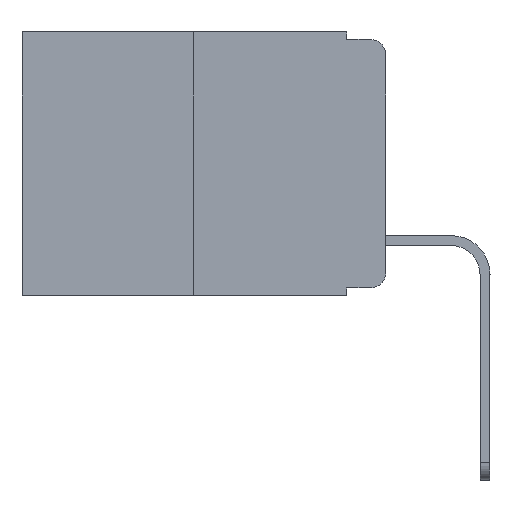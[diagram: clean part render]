
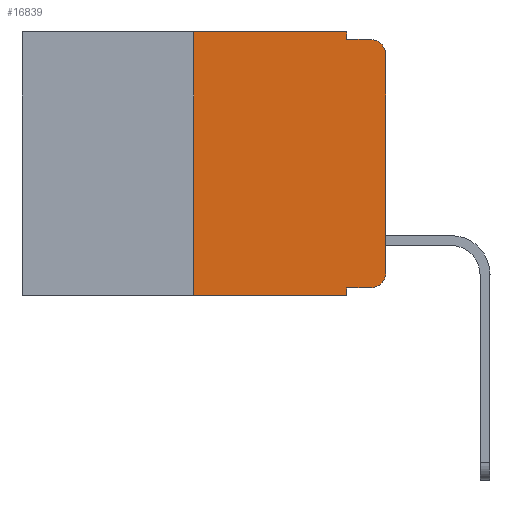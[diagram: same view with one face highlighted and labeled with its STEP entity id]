
A CAD part, left-side view. The second image highlights one B-rep face of the part: STEP entity #16839.
In plain terms, the highlighted planar face has unit normal (-1, 0, 0).
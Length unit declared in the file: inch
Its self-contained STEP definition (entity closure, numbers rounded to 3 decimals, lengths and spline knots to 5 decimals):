
#220 = ORIENTED_EDGE ( 'NONE', *, *, #14838, .F. ) ;
#288 = CARTESIAN_POINT ( 'NONE',  ( 0., 0., 0. ) ) ;
#631 = CARTESIAN_POINT ( 'NONE',  ( 0., 0.02, -0.333 ) ) ;
#777 = LINE ( 'NONE', #10494, #13447 ) ;
#1156 = EDGE_CURVE ( 'NONE', #20680, #15491, #10994, .T. ) ;
#1277 = LINE ( 'NONE', #19531, #8541 ) ;
#1590 = CARTESIAN_POINT ( 'NONE',  ( 0., 0.051, -0.343 ) ) ;
#1630 = CARTESIAN_POINT ( 'NONE',  ( 0., 0.02, -0.03 ) ) ;
#1922 = DIRECTION ( 'NONE',  ( 1., 0., 0. ) ) ;
#2115 = EDGE_CURVE ( 'NONE', #14703, #15491, #12535, .T. ) ;
#2386 = DIRECTION ( 'NONE',  ( 0., -1., 0. ) ) ;
#2475 = VERTEX_POINT ( 'NONE', #13945 ) ;
#2517 = DIRECTION ( 'NONE',  ( 0., 0., -1. ) ) ;
#3031 = AXIS2_PLACEMENT_3D ( 'NONE', #13689, #1922, #16672 ) ;
#3054 = DIRECTION ( 'NONE',  ( 0., 0., 1. ) ) ;
#3175 = DIRECTION ( 'NONE',  ( 0., 0., -1. ) ) ;
#3297 = EDGE_CURVE ( 'NONE', #20680, #5720, #17917, .T. ) ;
#3328 = CARTESIAN_POINT ( 'NONE',  ( 0., 0.473, 0. ) ) ;
#3386 = ORIENTED_EDGE ( 'NONE', *, *, #4852, .T. ) ;
#3617 = EDGE_CURVE ( 'NONE', #16788, #13889, #12475, .T. ) ;
#4710 = CIRCLE ( 'NONE', #8698, 0.02 ) ;
#4852 = EDGE_CURVE ( 'NONE', #5720, #16436, #14236, .T. ) ;
#5127 = PLANE ( 'NONE',  #3031 ) ;
#5217 = DIRECTION ( 'NONE',  ( 0., -1., 0. ) ) ;
#5290 = CARTESIAN_POINT ( 'NONE',  ( 0., 0.473, -0.343 ) ) ;
#5342 = EDGE_CURVE ( 'NONE', #11454, #16788, #777, .T. ) ;
#5442 = DIRECTION ( 'NONE',  ( 0., -1., 0. ) ) ;
#5638 = DIRECTION ( 'NONE',  ( -1., 0., 0. ) ) ;
#5720 = VERTEX_POINT ( 'NONE', #631 ) ;
#6202 = LINE ( 'NONE', #3328, #20914 ) ;
#6260 = EDGE_CURVE ( 'NONE', #2475, #11454, #6202, .T. ) ;
#6346 = EDGE_LOOP ( 'NONE', ( #14950, #16687, #19686, #13914, #16018, #220, #7639, #19569, #6549, #3386 ) ) ;
#6476 = VERTEX_POINT ( 'NONE', #9182 ) ;
#6549 = ORIENTED_EDGE ( 'NONE', *, *, #3297, .T. ) ;
#6559 = VECTOR ( 'NONE', #7291, 39.37008 ) ;
#6626 = VECTOR ( 'NONE', #16095, 39.37008 ) ;
#7291 = DIRECTION ( 'NONE',  ( 0., -1., 0. ) ) ;
#7639 = ORIENTED_EDGE ( 'NONE', *, *, #2115, .T. ) ;
#8345 = EDGE_CURVE ( 'NONE', #16436, #6476, #11234, .T. ) ;
#8446 = CARTESIAN_POINT ( 'NONE',  ( 0., 0.051, -0.333 ) ) ;
#8505 = CARTESIAN_POINT ( 'NONE',  ( 0., 0.02, -0.313 ) ) ;
#8541 = VECTOR ( 'NONE', #3054, 39.37008 ) ;
#8698 = AXIS2_PLACEMENT_3D ( 'NONE', #1630, #9328, #3175 ) ;
#9182 = CARTESIAN_POINT ( 'NONE',  ( 0., 0., -0.03 ) ) ;
#9328 = DIRECTION ( 'NONE',  ( -1., 0., 0. ) ) ;
#9680 = CARTESIAN_POINT ( 'NONE',  ( 0., 0.051, 0. ) ) ;
#10347 = AXIS2_PLACEMENT_3D ( 'NONE', #8505, #5638, #20269 ) ;
#10494 = CARTESIAN_POINT ( 'NONE',  ( 0., 0.051, 0. ) ) ;
#10994 = LINE ( 'NONE', #9680, #6626 ) ;
#11234 = LINE ( 'NONE', #288, #16653 ) ;
#11246 = FACE_OUTER_BOUND ( 'NONE', #6346, .T. ) ;
#11454 = VERTEX_POINT ( 'NONE', #17189 ) ;
#11861 = DIRECTION ( 'NONE',  ( 0., 0., 1. ) ) ;
#12475 = LINE ( 'NONE', #20470, #6559 ) ;
#12535 = LINE ( 'NONE', #5290, #19001 ) ;
#12569 = CARTESIAN_POINT ( 'NONE',  ( 0., 0., -0.313 ) ) ;
#13447 = VECTOR ( 'NONE', #2517, 39.37008 ) ;
#13579 = EDGE_CURVE ( 'NONE', #6476, #13889, #4710, .T. ) ;
#13689 = CARTESIAN_POINT ( 'NONE',  ( 0., 0.473, 0. ) ) ;
#13889 = VERTEX_POINT ( 'NONE', #20354 ) ;
#13914 = ORIENTED_EDGE ( 'NONE', *, *, #5342, .F. ) ;
#13945 = CARTESIAN_POINT ( 'NONE',  ( 0., 0.25, 0. ) ) ;
#14236 = CIRCLE ( 'NONE', #10347, 0.02 ) ;
#14703 = VERTEX_POINT ( 'NONE', #20906 ) ;
#14838 = EDGE_CURVE ( 'NONE', #14703, #2475, #1277, .T. ) ;
#14950 = ORIENTED_EDGE ( 'NONE', *, *, #8345, .T. ) ;
#14997 = CARTESIAN_POINT ( 'NONE',  ( 0., 0.051, -0.01 ) ) ;
#15491 = VERTEX_POINT ( 'NONE', #1590 ) ;
#16018 = ORIENTED_EDGE ( 'NONE', *, *, #6260, .F. ) ;
#16095 = DIRECTION ( 'NONE',  ( 0., 0., -1. ) ) ;
#16436 = VERTEX_POINT ( 'NONE', #12569 ) ;
#16653 = VECTOR ( 'NONE', #11861, 39.37008 ) ;
#16672 = DIRECTION ( 'NONE',  ( 0., 0., -1. ) ) ;
#16687 = ORIENTED_EDGE ( 'NONE', *, *, #13579, .T. ) ;
#16706 = CARTESIAN_POINT ( 'NONE',  ( 0., 0.051, -0.333 ) ) ;
#16788 = VERTEX_POINT ( 'NONE', #14997 ) ;
#16839 = ADVANCED_FACE ( 'NONE', ( #11246 ), #5127, .F. ) ;
#16881 = VECTOR ( 'NONE', #2386, 39.37008 ) ;
#17189 = CARTESIAN_POINT ( 'NONE',  ( 0., 0.051, 0. ) ) ;
#17917 = LINE ( 'NONE', #16706, #16881 ) ;
#19001 = VECTOR ( 'NONE', #5442, 39.37008 ) ;
#19531 = CARTESIAN_POINT ( 'NONE',  ( 0., 0.25, 0. ) ) ;
#19569 = ORIENTED_EDGE ( 'NONE', *, *, #1156, .F. ) ;
#19686 = ORIENTED_EDGE ( 'NONE', *, *, #3617, .F. ) ;
#20269 = DIRECTION ( 'NONE',  ( 0., 0., -1. ) ) ;
#20354 = CARTESIAN_POINT ( 'NONE',  ( 0., 0.02, -0.01 ) ) ;
#20470 = CARTESIAN_POINT ( 'NONE',  ( 0., 0.051, -0.01 ) ) ;
#20680 = VERTEX_POINT ( 'NONE', #8446 ) ;
#20906 = CARTESIAN_POINT ( 'NONE',  ( 0., 0.25, -0.343 ) ) ;
#20914 = VECTOR ( 'NONE', #5217, 39.37008 ) ;
